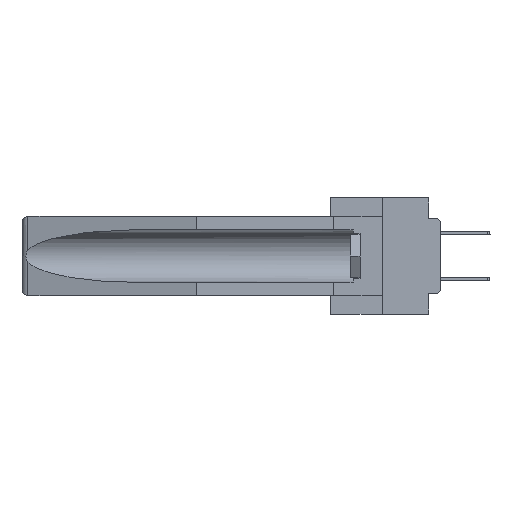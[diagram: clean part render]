
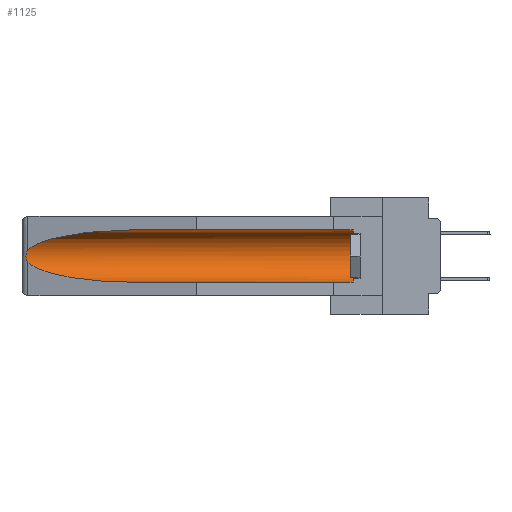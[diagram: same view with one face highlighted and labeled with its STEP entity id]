
A CAD part, left-side view. The second image highlights one B-rep face of the part: STEP entity #1125.
In plain terms, the highlighted cylindrical face has radius 2.857 mm (diameter 5.715 mm), a partial arc.
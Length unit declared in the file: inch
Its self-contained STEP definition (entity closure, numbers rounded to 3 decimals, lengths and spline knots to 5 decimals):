
#373 = CARTESIAN_POINT ( 'NONE',  ( 0.2673, 1.53269, -0.17917 ) ) ;
#446 = EDGE_CURVE ( 'NONE', #5549, #31225, #18360, .T. ) ;
#896 = CARTESIAN_POINT ( 'NONE',  ( 0.26537, 1.52718, -0.19328 ) ) ;
#1059 = CARTESIAN_POINT ( 'NONE',  ( 0.25451, 1.48313, -0.24835 ) ) ;
#1063 = AXIS2_PLACEMENT_3D ( 'NONE', #8349, #3639, #14309 ) ;
#1125 = ADVANCED_FACE ( 'NONE', ( #8710 ), #32762, .F. ) ;
#2398 = EDGE_CURVE ( 'NONE', #22701, #5549, #8515, .T. ) ;
#2701 = ORIENTED_EDGE ( 'NONE', *, *, #10513, .T. ) ;
#3639 = DIRECTION ( 'NONE',  ( 0., 1., 0. ) ) ;
#4287 = EDGE_CURVE ( 'NONE', #31659, #14405, #22864, .T. ) ;
#5092 = CARTESIAN_POINT ( 'NONE',  ( 0.2673, 1.5327, -0.16383 ) ) ;
#5406 = VECTOR ( 'NONE', #13740, 39.37008 ) ;
#5433 = CARTESIAN_POINT ( 'NONE',  ( 0.26537, 1.52718, -0.14972 ) ) ;
#5549 = VERTEX_POINT ( 'NONE', #23761 ) ;
#5826 = VECTOR ( 'NONE', #18370, 39.37008 ) ;
#6030 = CARTESIAN_POINT ( 'NONE',  ( 0.155, -0.30754, -0.059 ) ) ;
#6590 = CARTESIAN_POINT ( 'NONE',  ( 0.26537, 1.52718, -0.19328 ) ) ;
#7736 = CARTESIAN_POINT ( 'NONE',  ( 0.155, -0.30754, -0.284 ) ) ;
#7838 = CARTESIAN_POINT ( 'NONE',  ( 0.155, 0.126, -0.1715 ) ) ;
#7874 = CARTESIAN_POINT ( 'NONE',  ( 0.26655, 1.53094, -0.18657 ) ) ;
#8228 = CARTESIAN_POINT ( 'NONE',  ( 0.2675, 1.53308, -0.16763 ) ) ;
#8346 = DIRECTION ( 'NONE',  ( 0., 0., 1. ) ) ;
#8349 = CARTESIAN_POINT ( 'NONE',  ( 0.155, -0.30754, -0.1715 ) ) ;
#8515 =( BOUNDED_CURVE ( )  B_SPLINE_CURVE ( 3, ( #9808, #28639, #17996, #31580 ),
 .UNSPECIFIED., .F., .F. ) 
 B_SPLINE_CURVE_WITH_KNOTS ( ( 4, 4 ),
 ( 4.71239, 6.08839 ),
 .UNSPECIFIED. ) 
 CURVE ( )  GEOMETRIC_REPRESENTATION_ITEM ( )  RATIONAL_B_SPLINE_CURVE ( ( 1., 0.848, 0.848, 1. ) ) 
 REPRESENTATION_ITEM ( '' )  );
#8710 = FACE_OUTER_BOUND ( 'NONE', #29520, .T. ) ;
#9808 = CARTESIAN_POINT ( 'NONE',  ( 0.155, 1.07973, -0.059 ) ) ;
#10507 = CARTESIAN_POINT ( 'NONE',  ( 0.26597, 1.52961, -0.15275 ) ) ;
#10513 = EDGE_CURVE ( 'NONE', #31225, #13077, #26345, .T. ) ;
#11025 = CARTESIAN_POINT ( 'NONE',  ( 0.26597, 1.5296, -0.19026 ) ) ;
#11257 = ORIENTED_EDGE ( 'NONE', *, *, #11344, .F. ) ;
#11344 = EDGE_CURVE ( 'NONE', #31659, #13077, #20998, .T. ) ;
#11896 = ORIENTED_EDGE ( 'NONE', *, *, #2398, .T. ) ;
#13077 = VERTEX_POINT ( 'NONE', #34030 ) ;
#13134 = CARTESIAN_POINT ( 'NONE',  ( 0.26537, 1.52718, -0.19328 ) ) ;
#13740 = DIRECTION ( 'NONE',  ( 0., 1., 0. ) ) ;
#14309 = DIRECTION ( 'NONE',  ( 0., 0., 1. ) ) ;
#14405 = VERTEX_POINT ( 'NONE', #23754 ) ;
#15277 = EDGE_CURVE ( 'NONE', #14405, #22701, #16873, .T. ) ;
#15685 = AXIS2_PLACEMENT_3D ( 'NONE', #7838, #32240, #8346 ) ;
#16269 = CARTESIAN_POINT ( 'NONE',  ( 0.2675, 1.53308, -0.17534 ) ) ;
#16873 = LINE ( 'NONE', #6030, #5406 ) ;
#17996 = CARTESIAN_POINT ( 'NONE',  ( 0.25451, 1.48313, -0.09465 ) ) ;
#18360 = B_SPLINE_CURVE_WITH_KNOTS ( 'NONE', 3,
 ( #5433, #10507, #32110, #5092, #8228, #16269, #373, #7874, #11025, #13134 ),
 .UNSPECIFIED., .F., .F.,
 ( 4, 2, 2, 2, 4 ),
 ( 0., 0.00029, 0.00058, 0.00087, 0.00117 ),
 .UNSPECIFIED. ) ;
#18370 = DIRECTION ( 'NONE',  ( 0., 1., 0. ) ) ;
#20998 = LINE ( 'NONE', #7736, #5826 ) ;
#21630 = ORIENTED_EDGE ( 'NONE', *, *, #15277, .T. ) ;
#22233 = ORIENTED_EDGE ( 'NONE', *, *, #446, .T. ) ;
#22701 = VERTEX_POINT ( 'NONE', #29716 ) ;
#22864 = CIRCLE ( 'NONE', #15685, 0.1125 ) ;
#23754 = CARTESIAN_POINT ( 'NONE',  ( 0.155, 0.126, -0.059 ) ) ;
#23761 = CARTESIAN_POINT ( 'NONE',  ( 0.26537, 1.52718, -0.14972 ) ) ;
#26345 =( BOUNDED_CURVE ( )  B_SPLINE_CURVE ( 3, ( #896, #1059, #27382, #30358 ),
 .UNSPECIFIED., .F., .F. ) 
 B_SPLINE_CURVE_WITH_KNOTS ( ( 4, 4 ),
 ( 0.1948, 1.5708 ),
 .UNSPECIFIED. ) 
 CURVE ( )  GEOMETRIC_REPRESENTATION_ITEM ( )  RATIONAL_B_SPLINE_CURVE ( ( 1., 0.848, 0.848, 1. ) ) 
 REPRESENTATION_ITEM ( '' )  );
#27382 = CARTESIAN_POINT ( 'NONE',  ( 0.21114, 1.30732, -0.284 ) ) ;
#27540 = ORIENTED_EDGE ( 'NONE', *, *, #4287, .T. ) ;
#28639 = CARTESIAN_POINT ( 'NONE',  ( 0.21114, 1.30732, -0.059 ) ) ;
#29520 = EDGE_LOOP ( 'NONE', ( #11896, #22233, #2701, #11257, #27540, #21630 ) ) ;
#29716 = CARTESIAN_POINT ( 'NONE',  ( 0.155, 1.07973, -0.059 ) ) ;
#30358 = CARTESIAN_POINT ( 'NONE',  ( 0.155, 1.07973, -0.284 ) ) ;
#31225 = VERTEX_POINT ( 'NONE', #6590 ) ;
#31580 = CARTESIAN_POINT ( 'NONE',  ( 0.26537, 1.52718, -0.14972 ) ) ;
#31659 = VERTEX_POINT ( 'NONE', #33430 ) ;
#32110 = CARTESIAN_POINT ( 'NONE',  ( 0.26654, 1.53092, -0.15636 ) ) ;
#32240 = DIRECTION ( 'NONE',  ( 0., -1., 0. ) ) ;
#32762 = CYLINDRICAL_SURFACE ( 'NONE', #1063, 0.1125 ) ;
#33430 = CARTESIAN_POINT ( 'NONE',  ( 0.155, 0.126, -0.284 ) ) ;
#34030 = CARTESIAN_POINT ( 'NONE',  ( 0.155, 1.07973, -0.284 ) ) ;
